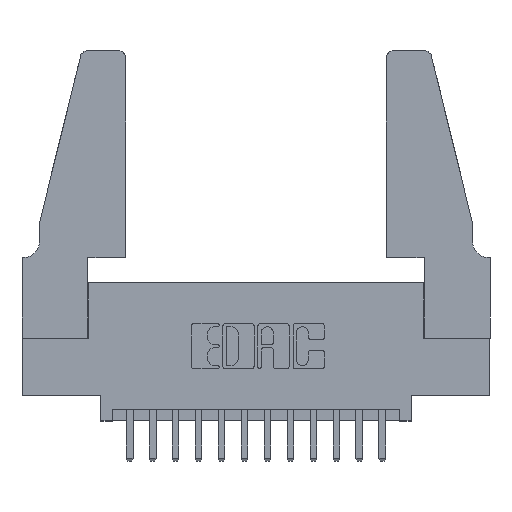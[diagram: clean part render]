
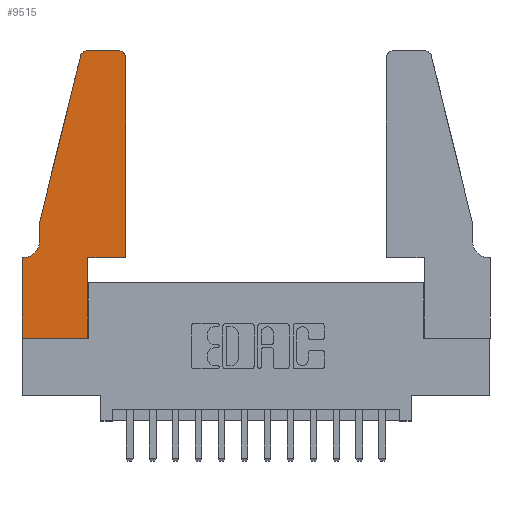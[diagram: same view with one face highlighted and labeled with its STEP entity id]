
A CAD part, top view. The second image highlights one B-rep face of the part: STEP entity #9515.
In plain terms, the highlighted planar face has unit normal (0, 0, 1).
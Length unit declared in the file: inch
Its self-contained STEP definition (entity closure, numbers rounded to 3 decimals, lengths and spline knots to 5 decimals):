
#126 = ORIENTED_EDGE ( 'NONE', *, *, #4946, .T. ) ;
#219 = DIRECTION ( 'NONE',  ( 1., 0., 0. ) ) ;
#561 = DIRECTION ( 'NONE',  ( 1., 0., 0. ) ) ;
#578 = CARTESIAN_POINT ( 'NONE',  ( 0.25487, 1.22718, 0.37 ) ) ;
#737 = DIRECTION ( 'NONE',  ( -1., 0., 0. ) ) ;
#817 = DIRECTION ( 'NONE',  ( 0., -1., 0. ) ) ;
#1075 = DIRECTION ( 'NONE',  ( -1., 0., 0. ) ) ;
#1165 = CARTESIAN_POINT ( 'NONE',  ( 0.2865, 0.35, 0.37 ) ) ;
#1169 = CARTESIAN_POINT ( 'NONE',  ( 0.0055, 0.42, 0.37 ) ) ;
#1289 = DIRECTION ( 'NONE',  ( 0., 0., -1. ) ) ;
#1421 = EDGE_CURVE ( 'NONE', #7183, #10334, #4651, .T. ) ;
#1457 = ORIENTED_EDGE ( 'NONE', *, *, #7494, .T. ) ;
#1638 = CARTESIAN_POINT ( 'NONE',  ( 0.4505, 0.35, 0.37 ) ) ;
#1674 = LINE ( 'NONE', #14047, #13514 ) ;
#1789 = CARTESIAN_POINT ( 'NONE',  ( 0.0755, 0.5, 0.37 ) ) ;
#2256 = VECTOR ( 'NONE', #737, 39.37008 ) ;
#2266 = ORIENTED_EDGE ( 'NONE', *, *, #15481, .T. ) ;
#2353 = DIRECTION ( 'NONE',  ( 1., 0., 0. ) ) ;
#2446 = VERTEX_POINT ( 'NONE', #11141 ) ;
#2458 = VERTEX_POINT ( 'NONE', #11534 ) ;
#2662 = VERTEX_POINT ( 'NONE', #1638 ) ;
#2709 = EDGE_CURVE ( 'NONE', #5241, #10259, #15775, .T. ) ;
#2850 = CARTESIAN_POINT ( 'NONE',  ( 0.2865, 0.35, 0.37 ) ) ;
#2873 = DIRECTION ( 'NONE',  ( 0., -1., 0. ) ) ;
#2942 = CARTESIAN_POINT ( 'NONE',  ( 0.0055, 0.35, 0.37 ) ) ;
#2991 = ORIENTED_EDGE ( 'NONE', *, *, #5076, .T. ) ;
#3045 = CARTESIAN_POINT ( 'NONE',  ( 0., 0.35, 0.37 ) ) ;
#3164 = DIRECTION ( 'NONE',  ( 0., 0., 1. ) ) ;
#3307 = VECTOR ( 'NONE', #817, 39.37008 ) ;
#3324 = LINE ( 'NONE', #1165, #13030 ) ;
#3427 = EDGE_CURVE ( 'NONE', #11327, #2446, #10390, .T. ) ;
#3759 = VERTEX_POINT ( 'NONE', #1789 ) ;
#4261 = LINE ( 'NONE', #10868, #13949 ) ;
#4310 = CARTESIAN_POINT ( 'NONE',  ( 0.2865, 0., 0.37 ) ) ;
#4500 = ORIENTED_EDGE ( 'NONE', *, *, #2709, .T. ) ;
#4597 = VECTOR ( 'NONE', #6164, 39.37008 ) ;
#4651 = CIRCLE ( 'NONE', #11796, 0.03 ) ;
#4703 = LINE ( 'NONE', #6636, #7956 ) ;
#4856 = DIRECTION ( 'NONE',  ( 1., 0., 0. ) ) ;
#4946 = EDGE_CURVE ( 'NONE', #9828, #2458, #6533, .T. ) ;
#5076 = EDGE_CURVE ( 'NONE', #6643, #2662, #4261, .T. ) ;
#5241 = VERTEX_POINT ( 'NONE', #9929 ) ;
#6164 = DIRECTION ( 'NONE',  ( 0., 1., 0. ) ) ;
#6458 = EDGE_CURVE ( 'NONE', #2662, #11327, #7835, .T. ) ;
#6533 = LINE ( 'NONE', #15460, #3307 ) ;
#6537 = AXIS2_PLACEMENT_3D ( 'NONE', #9715, #12131, #4856 ) ;
#6635 = LINE ( 'NONE', #8966, #13106 ) ;
#6636 = CARTESIAN_POINT ( 'NONE',  ( 0.0755, 0.5, 0.37 ) ) ;
#6643 = VERTEX_POINT ( 'NONE', #2850 ) ;
#7116 = ORIENTED_EDGE ( 'NONE', *, *, #12164, .T. ) ;
#7183 = VERTEX_POINT ( 'NONE', #7467 ) ;
#7249 = PLANE ( 'NONE',  #6537 ) ;
#7298 = CARTESIAN_POINT ( 'NONE',  ( 0.284, 1.22, 0.37 ) ) ;
#7322 = DIRECTION ( 'NONE',  ( 0., 1., 0. ) ) ;
#7467 = CARTESIAN_POINT ( 'NONE',  ( 0.284, 1.25, 0.37 ) ) ;
#7494 = EDGE_CURVE ( 'NONE', #2446, #7183, #11958, .T. ) ;
#7835 = LINE ( 'NONE', #9781, #4597 ) ;
#7932 = EDGE_CURVE ( 'NONE', #3759, #5241, #6635, .T. ) ;
#7956 = VECTOR ( 'NONE', #12695, 39.37008 ) ;
#8072 = EDGE_CURVE ( 'NONE', #2458, #8594, #10799, .T. ) ;
#8594 = VERTEX_POINT ( 'NONE', #4310 ) ;
#8776 = DIRECTION ( 'NONE',  ( 0., 0., 1. ) ) ;
#8927 = FACE_OUTER_BOUND ( 'NONE', #10234, .T. ) ;
#8966 = CARTESIAN_POINT ( 'NONE',  ( 0.0755, 0.5, 0.37 ) ) ;
#9407 = ORIENTED_EDGE ( 'NONE', *, *, #1421, .T. ) ;
#9515 = ADVANCED_FACE ( 'NONE', ( #8927 ), #7249, .T. ) ;
#9694 = ORIENTED_EDGE ( 'NONE', *, *, #8072, .T. ) ;
#9715 = CARTESIAN_POINT ( 'NONE',  ( 0., 0.35, 0.37 ) ) ;
#9781 = CARTESIAN_POINT ( 'NONE',  ( 0.4505, 0.35, 0.37 ) ) ;
#9828 = VERTEX_POINT ( 'NONE', #3045 ) ;
#9929 = CARTESIAN_POINT ( 'NONE',  ( 0.0755, 0.42, 0.37 ) ) ;
#10234 = EDGE_LOOP ( 'NONE', ( #1457, #9407, #2266, #14167, #4500, #11445, #126, #9694, #7116, #2991, #15741, #11552 ) ) ;
#10259 = VERTEX_POINT ( 'NONE', #2942 ) ;
#10334 = VERTEX_POINT ( 'NONE', #578 ) ;
#10390 = CIRCLE ( 'NONE', #15025, 0.03 ) ;
#10421 = CARTESIAN_POINT ( 'NONE',  ( 0., 0., 0.37 ) ) ;
#10429 = CARTESIAN_POINT ( 'NONE',  ( 0.4205, 1.22, 0.37 ) ) ;
#10799 = LINE ( 'NONE', #10421, #14049 ) ;
#10868 = CARTESIAN_POINT ( 'NONE',  ( 0.4505, 0.35, 0.37 ) ) ;
#11141 = CARTESIAN_POINT ( 'NONE',  ( 0.4205, 1.25, 0.37 ) ) ;
#11327 = VERTEX_POINT ( 'NONE', #13602 ) ;
#11445 = ORIENTED_EDGE ( 'NONE', *, *, #14027, .T. ) ;
#11462 = DIRECTION ( 'NONE',  ( 1., 0., 0. ) ) ;
#11534 = CARTESIAN_POINT ( 'NONE',  ( 0., 0., 0.37 ) ) ;
#11552 = ORIENTED_EDGE ( 'NONE', *, *, #3427, .T. ) ;
#11796 = AXIS2_PLACEMENT_3D ( 'NONE', #7298, #3164, #219 ) ;
#11958 = LINE ( 'NONE', #15400, #2256 ) ;
#12131 = DIRECTION ( 'NONE',  ( 0., 0., 1. ) ) ;
#12164 = EDGE_CURVE ( 'NONE', #8594, #6643, #3324, .T. ) ;
#12695 = DIRECTION ( 'NONE',  ( -0.239, -0.971, 0. ) ) ;
#12825 = DIRECTION ( 'NONE',  ( -1., 0., 0. ) ) ;
#13030 = VECTOR ( 'NONE', #7322, 39.37008 ) ;
#13106 = VECTOR ( 'NONE', #2873, 39.37008 ) ;
#13252 = AXIS2_PLACEMENT_3D ( 'NONE', #1169, #1289, #1075 ) ;
#13514 = VECTOR ( 'NONE', #12825, 39.37008 ) ;
#13602 = CARTESIAN_POINT ( 'NONE',  ( 0.4505, 1.22, 0.37 ) ) ;
#13949 = VECTOR ( 'NONE', #2353, 39.37008 ) ;
#14027 = EDGE_CURVE ( 'NONE', #10259, #9828, #1674, .T. ) ;
#14047 = CARTESIAN_POINT ( 'NONE',  ( 0.0755, 0.35, 0.37 ) ) ;
#14049 = VECTOR ( 'NONE', #561, 39.37008 ) ;
#14167 = ORIENTED_EDGE ( 'NONE', *, *, #7932, .T. ) ;
#15025 = AXIS2_PLACEMENT_3D ( 'NONE', #10429, #8776, #11462 ) ;
#15400 = CARTESIAN_POINT ( 'NONE',  ( 0.2605, 1.25, 0.37 ) ) ;
#15460 = CARTESIAN_POINT ( 'NONE',  ( 0., 0., 0.37 ) ) ;
#15481 = EDGE_CURVE ( 'NONE', #10334, #3759, #4703, .T. ) ;
#15741 = ORIENTED_EDGE ( 'NONE', *, *, #6458, .T. ) ;
#15775 = CIRCLE ( 'NONE', #13252, 0.07 ) ;
